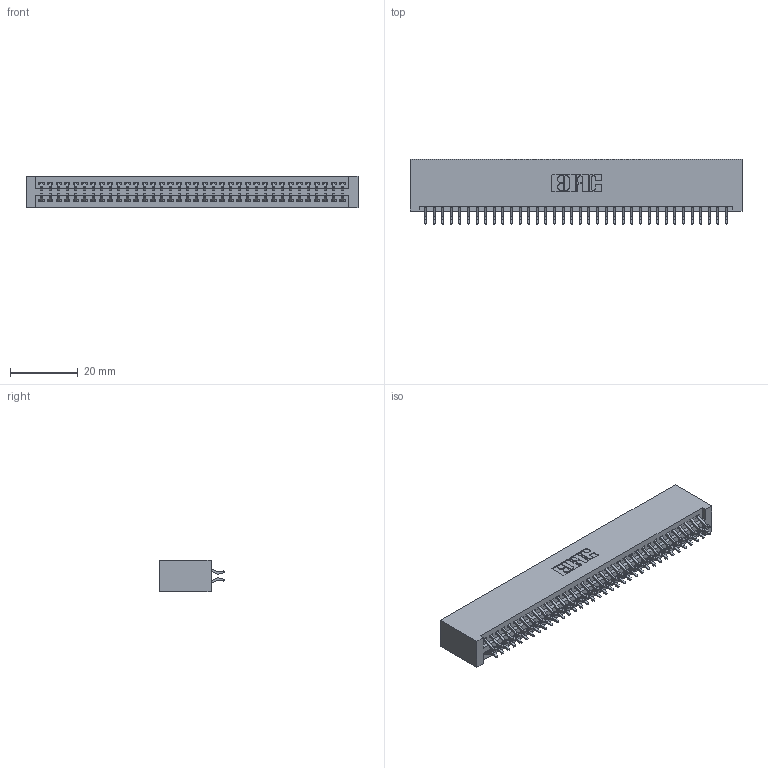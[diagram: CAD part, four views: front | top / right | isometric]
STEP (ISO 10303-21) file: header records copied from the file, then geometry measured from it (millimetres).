
FILE_DESCRIPTION (( 'STEP AP203' ), '1' );
FILE_NAME ('395-072-556-201.STEP', '2018-11-27T15:14:02', ( '' ), ( '' ), 'SwSTEP 2.0', 'SolidWorks 2016', '' );
FILE_SCHEMA (( 'CONFIG_CONTROL_DESIGN' ));
Length unit declared in the file: inch
Products named in the file (3): 395-072-556-201; 345-292-001_556 Tail; 345 Part_No Mounting Lugs
Assembly tree (73 placements, depth 2):
  395-072-556-201
    345 Part_No Mounting Lugs
    345-292-001_556 Tail  x72
Bounding box: 98.04 x 19.24 x 9.4 mm (x, y, z)
Volume: 10081.5 mm3; surface area: 15026.1 mm2
Topology: 73 solids, 73 shells, 4150 faces, 12341 edges, 8130 vertices
Faces by surface type: plane 2740, cylinder 1410
Entity records: 28997 total; most frequent: CARTESIAN_POINT 4880, ORIENTED_EDGE 4802, DIRECTION 4293, EDGE_CURVE 2401, LINE 2125, VECTOR 2125, VERTEX_POINT 1598, AXIS2_PLACEMENT_3D 1084
